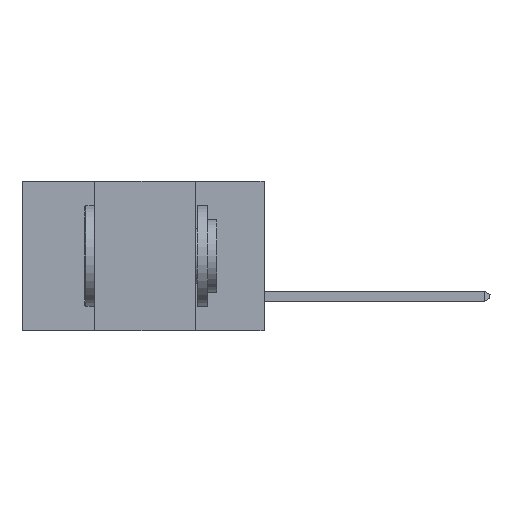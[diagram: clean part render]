
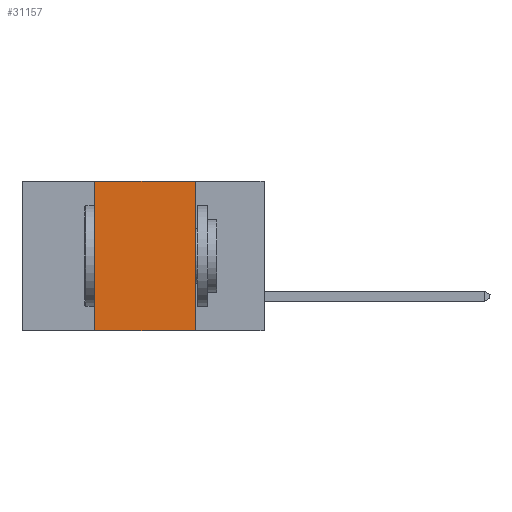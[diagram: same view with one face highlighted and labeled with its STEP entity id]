
A CAD part, left-side view. The second image highlights one B-rep face of the part: STEP entity #31157.
In plain terms, the highlighted planar face has unit normal (-1, 0, 0).
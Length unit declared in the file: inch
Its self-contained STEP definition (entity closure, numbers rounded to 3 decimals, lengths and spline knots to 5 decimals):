
#374 = VERTEX_POINT ( 'NONE', #1283 ) ;
#1283 = CARTESIAN_POINT ( 'NONE',  ( 0., 0.17, 0. ) ) ;
#1466 = EDGE_LOOP ( 'NONE', ( #18965, #11808, #3576, #24573 ) ) ;
#2221 = CARTESIAN_POINT ( 'NONE',  ( 0., 0.6, -0.37 ) ) ;
#3026 = EDGE_CURVE ( 'NONE', #29482, #25819, #9431, .T. ) ;
#3452 = VECTOR ( 'NONE', #10750, 39.37008 ) ;
#3576 = ORIENTED_EDGE ( 'NONE', *, *, #3026, .F. ) ;
#5066 = VECTOR ( 'NONE', #20827, 39.37008 ) ;
#7429 = DIRECTION ( 'NONE',  ( 1., 0., 0. ) ) ;
#8411 = EDGE_CURVE ( 'NONE', #29482, #30334, #15703, .T. ) ;
#8935 = EDGE_CURVE ( 'NONE', #374, #30334, #29437, .T. ) ;
#9431 = LINE ( 'NONE', #15879, #5066 ) ;
#9990 = CARTESIAN_POINT ( 'NONE',  ( 0., 0.42, -0.37 ) ) ;
#10229 = EDGE_CURVE ( 'NONE', #25819, #374, #12451, .T. ) ;
#10750 = DIRECTION ( 'NONE',  ( 0., 0., -1. ) ) ;
#11808 = ORIENTED_EDGE ( 'NONE', *, *, #10229, .F. ) ;
#12451 = LINE ( 'NONE', #28533, #28536 ) ;
#15703 = LINE ( 'NONE', #2221, #31795 ) ;
#15879 = CARTESIAN_POINT ( 'NONE',  ( 0., 0.42, 0. ) ) ;
#16034 = DIRECTION ( 'NONE',  ( 0., -1., 0. ) ) ;
#16156 = CARTESIAN_POINT ( 'NONE',  ( 0., 0.17, 0. ) ) ;
#17753 = DIRECTION ( 'NONE',  ( 0., -1., 0. ) ) ;
#17777 = CARTESIAN_POINT ( 'NONE',  ( 0., 0.17, -0.37 ) ) ;
#18783 = AXIS2_PLACEMENT_3D ( 'NONE', #32179, #7429, #19660 ) ;
#18965 = ORIENTED_EDGE ( 'NONE', *, *, #8935, .F. ) ;
#19660 = DIRECTION ( 'NONE',  ( 0., 0., -1. ) ) ;
#20827 = DIRECTION ( 'NONE',  ( 0., 0., 1. ) ) ;
#24573 = ORIENTED_EDGE ( 'NONE', *, *, #8411, .T. ) ;
#25819 = VERTEX_POINT ( 'NONE', #26880 ) ;
#26880 = CARTESIAN_POINT ( 'NONE',  ( 0., 0.42, 0. ) ) ;
#28533 = CARTESIAN_POINT ( 'NONE',  ( 0., 0.6, 0. ) ) ;
#28536 = VECTOR ( 'NONE', #16034, 39.37008 ) ;
#28873 = FACE_OUTER_BOUND ( 'NONE', #1466, .T. ) ;
#29437 = LINE ( 'NONE', #16156, #3452 ) ;
#29482 = VERTEX_POINT ( 'NONE', #9990 ) ;
#30334 = VERTEX_POINT ( 'NONE', #17777 ) ;
#31157 = ADVANCED_FACE ( 'NONE', ( #28873 ), #32288, .F. ) ;
#31795 = VECTOR ( 'NONE', #17753, 39.37008 ) ;
#32179 = CARTESIAN_POINT ( 'NONE',  ( 0., 0.6, 0. ) ) ;
#32288 = PLANE ( 'NONE',  #18783 ) ;
